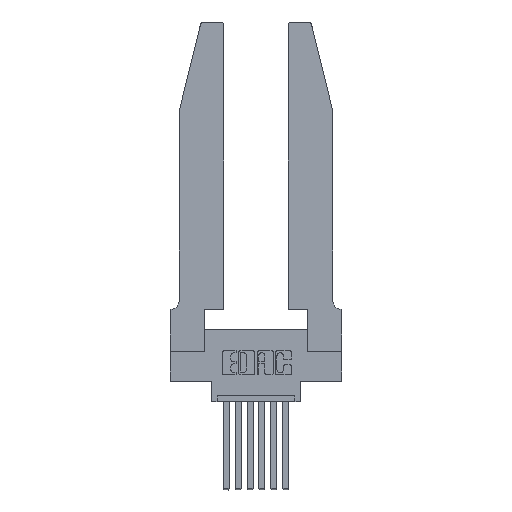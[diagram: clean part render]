
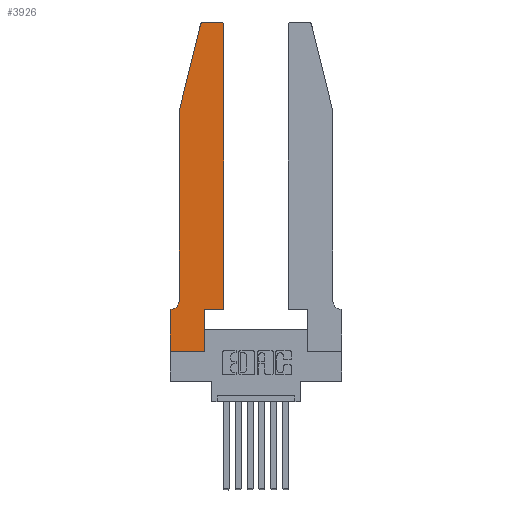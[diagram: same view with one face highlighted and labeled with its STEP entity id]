
A CAD part, top view. The second image highlights one B-rep face of the part: STEP entity #3926.
In plain terms, the highlighted planar face has unit normal (0, 0, 1).
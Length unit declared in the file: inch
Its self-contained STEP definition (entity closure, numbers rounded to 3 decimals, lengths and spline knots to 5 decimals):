
#338 = DIRECTION ( 'NONE',  ( 0., 1., 0. ) ) ;
#465 = ORIENTED_EDGE ( 'NONE', *, *, #9877, .T. ) ;
#530 = CARTESIAN_POINT ( 'NONE',  ( 0.25487, 2.72718, 0.37 ) ) ;
#577 = VECTOR ( 'NONE', #11728, 39.37008 ) ;
#966 = DIRECTION ( 'NONE',  ( 1., 0., 0. ) ) ;
#974 = LINE ( 'NONE', #13848, #13574 ) ;
#1001 = EDGE_LOOP ( 'NONE', ( #7670, #6394, #12149, #5676, #9165, #8569, #6731, #13480, #465, #3043, #10294, #7103 ) ) ;
#1427 = VECTOR ( 'NONE', #12442, 39.37008 ) ;
#1522 = CARTESIAN_POINT ( 'NONE',  ( 0.2865, 0.35, 0.37 ) ) ;
#1587 = VERTEX_POINT ( 'NONE', #5933 ) ;
#1588 = VERTEX_POINT ( 'NONE', #9329 ) ;
#1752 = VERTEX_POINT ( 'NONE', #9555 ) ;
#2120 = AXIS2_PLACEMENT_3D ( 'NONE', #5850, #12301, #6760 ) ;
#2475 = DIRECTION ( 'NONE',  ( 0., 0., 1. ) ) ;
#2496 = CARTESIAN_POINT ( 'NONE',  ( 0.0755, 2., 0.37 ) ) ;
#2511 = CARTESIAN_POINT ( 'NONE',  ( 0.0755, 0.42, 0.37 ) ) ;
#2732 = EDGE_CURVE ( 'NONE', #7018, #10086, #8358, .T. ) ;
#2941 = VERTEX_POINT ( 'NONE', #6949 ) ;
#3043 = ORIENTED_EDGE ( 'NONE', *, *, #10945, .T. ) ;
#3095 = AXIS2_PLACEMENT_3D ( 'NONE', #6288, #5360, #966 ) ;
#3501 = DIRECTION ( 'NONE',  ( 0., -1., 0. ) ) ;
#3838 = CARTESIAN_POINT ( 'NONE',  ( 0.2865, 0.35, 0.37 ) ) ;
#3926 = ADVANCED_FACE ( 'NONE', ( #5076 ), #10661, .T. ) ;
#3950 = VECTOR ( 'NONE', #4097, 39.37008 ) ;
#4097 = DIRECTION ( 'NONE',  ( 0., -1., 0. ) ) ;
#4111 = EDGE_CURVE ( 'NONE', #4497, #4289, #11356, .T. ) ;
#4289 = VERTEX_POINT ( 'NONE', #7799 ) ;
#4497 = VERTEX_POINT ( 'NONE', #2511 ) ;
#4593 = CARTESIAN_POINT ( 'NONE',  ( 0.284, 2.75, 0.37 ) ) ;
#4658 = CARTESIAN_POINT ( 'NONE',  ( 0.4205, 2.72, 0.37 ) ) ;
#4994 = DIRECTION ( 'NONE',  ( -1., 0., 0. ) ) ;
#5076 = FACE_OUTER_BOUND ( 'NONE', #1001, .T. ) ;
#5276 = CARTESIAN_POINT ( 'NONE',  ( 0., 0., 0.37 ) ) ;
#5311 = VECTOR ( 'NONE', #3501, 39.37008 ) ;
#5334 = VERTEX_POINT ( 'NONE', #3838 ) ;
#5360 = DIRECTION ( 'NONE',  ( 0., 0., 1. ) ) ;
#5568 = EDGE_CURVE ( 'NONE', #9836, #9139, #8239, .T. ) ;
#5650 = DIRECTION ( 'NONE',  ( 1., 0., 0. ) ) ;
#5676 = ORIENTED_EDGE ( 'NONE', *, *, #7313, .T. ) ;
#5850 = CARTESIAN_POINT ( 'NONE',  ( 0.0055, 0.42, 0.37 ) ) ;
#5933 = CARTESIAN_POINT ( 'NONE',  ( 0., 0.35, 0.37 ) ) ;
#6051 = VECTOR ( 'NONE', #13645, 39.37008 ) ;
#6288 = CARTESIAN_POINT ( 'NONE',  ( 0., 0.35, 0.37 ) ) ;
#6394 = ORIENTED_EDGE ( 'NONE', *, *, #11330, .T. ) ;
#6709 = DIRECTION ( 'NONE',  ( 1., 0., 0. ) ) ;
#6722 = LINE ( 'NONE', #10276, #1427 ) ;
#6731 = ORIENTED_EDGE ( 'NONE', *, *, #7229, .T. ) ;
#6760 = DIRECTION ( 'NONE',  ( -1., 0., 0. ) ) ;
#6948 = CARTESIAN_POINT ( 'NONE',  ( 0.4205, 2.75, 0.37 ) ) ;
#6949 = CARTESIAN_POINT ( 'NONE',  ( 0., 0., 0.37 ) ) ;
#7018 = VERTEX_POINT ( 'NONE', #8177 ) ;
#7103 = ORIENTED_EDGE ( 'NONE', *, *, #10800, .T. ) ;
#7141 = LINE ( 'NONE', #1522, #8795 ) ;
#7229 = EDGE_CURVE ( 'NONE', #1587, #2941, #9677, .T. ) ;
#7260 = CARTESIAN_POINT ( 'NONE',  ( 0.4505, 0.35, 0.37 ) ) ;
#7313 = EDGE_CURVE ( 'NONE', #1588, #4497, #8182, .T. ) ;
#7504 = VERTEX_POINT ( 'NONE', #530 ) ;
#7670 = ORIENTED_EDGE ( 'NONE', *, *, #5568, .T. ) ;
#7765 = DIRECTION ( 'NONE',  ( 0., 0., 1. ) ) ;
#7799 = CARTESIAN_POINT ( 'NONE',  ( 0.0055, 0.35, 0.37 ) ) ;
#7951 = VECTOR ( 'NONE', #5650, 39.37008 ) ;
#8062 = VECTOR ( 'NONE', #4994, 39.37008 ) ;
#8177 = CARTESIAN_POINT ( 'NONE',  ( 0.4505, 0.35, 0.37 ) ) ;
#8182 = LINE ( 'NONE', #2496, #5311 ) ;
#8239 = LINE ( 'NONE', #11402, #8062 ) ;
#8358 = LINE ( 'NONE', #7260, #577 ) ;
#8474 = CARTESIAN_POINT ( 'NONE',  ( 0.4505, 2.72, 0.37 ) ) ;
#8569 = ORIENTED_EDGE ( 'NONE', *, *, #13128, .T. ) ;
#8607 = CIRCLE ( 'NONE', #12874, 0.03 ) ;
#8795 = VECTOR ( 'NONE', #338, 39.37008 ) ;
#8949 = CARTESIAN_POINT ( 'NONE',  ( 0., 0., 0.37 ) ) ;
#9139 = VERTEX_POINT ( 'NONE', #4593 ) ;
#9165 = ORIENTED_EDGE ( 'NONE', *, *, #4111, .T. ) ;
#9255 = LINE ( 'NONE', #12581, #6051 ) ;
#9329 = CARTESIAN_POINT ( 'NONE',  ( 0.0755, 2., 0.37 ) ) ;
#9555 = CARTESIAN_POINT ( 'NONE',  ( 0.2865, 0., 0.37 ) ) ;
#9677 = LINE ( 'NONE', #5276, #3950 ) ;
#9836 = VERTEX_POINT ( 'NONE', #6948 ) ;
#9877 = EDGE_CURVE ( 'NONE', #1752, #5334, #7141, .T. ) ;
#9920 = AXIS2_PLACEMENT_3D ( 'NONE', #13400, #2475, #6709 ) ;
#9926 = DIRECTION ( 'NONE',  ( 1., 0., 0. ) ) ;
#9951 = CIRCLE ( 'NONE', #9920, 0.03 ) ;
#10086 = VERTEX_POINT ( 'NONE', #8474 ) ;
#10276 = CARTESIAN_POINT ( 'NONE',  ( 0.0755, 0.35, 0.37 ) ) ;
#10286 = EDGE_CURVE ( 'NONE', #2941, #1752, #12412, .T. ) ;
#10294 = ORIENTED_EDGE ( 'NONE', *, *, #2732, .T. ) ;
#10661 = PLANE ( 'NONE',  #3095 ) ;
#10800 = EDGE_CURVE ( 'NONE', #10086, #9836, #8607, .T. ) ;
#10945 = EDGE_CURVE ( 'NONE', #5334, #7018, #974, .T. ) ;
#11330 = EDGE_CURVE ( 'NONE', #9139, #7504, #9951, .T. ) ;
#11356 = CIRCLE ( 'NONE', #2120, 0.07 ) ;
#11402 = CARTESIAN_POINT ( 'NONE',  ( 0.2605, 2.75, 0.37 ) ) ;
#11728 = DIRECTION ( 'NONE',  ( 0., 1., 0. ) ) ;
#12149 = ORIENTED_EDGE ( 'NONE', *, *, #13210, .T. ) ;
#12301 = DIRECTION ( 'NONE',  ( 0., 0., -1. ) ) ;
#12412 = LINE ( 'NONE', #8949, #7951 ) ;
#12442 = DIRECTION ( 'NONE',  ( -1., 0., 0. ) ) ;
#12581 = CARTESIAN_POINT ( 'NONE',  ( 0.0755, 2., 0.37 ) ) ;
#12874 = AXIS2_PLACEMENT_3D ( 'NONE', #4658, #7765, #9926 ) ;
#13128 = EDGE_CURVE ( 'NONE', #4289, #1587, #6722, .T. ) ;
#13210 = EDGE_CURVE ( 'NONE', #7504, #1588, #9255, .T. ) ;
#13400 = CARTESIAN_POINT ( 'NONE',  ( 0.284, 2.72, 0.37 ) ) ;
#13480 = ORIENTED_EDGE ( 'NONE', *, *, #10286, .T. ) ;
#13574 = VECTOR ( 'NONE', #13661, 39.37008 ) ;
#13645 = DIRECTION ( 'NONE',  ( -0.239, -0.971, 0. ) ) ;
#13661 = DIRECTION ( 'NONE',  ( 1., 0., 0. ) ) ;
#13848 = CARTESIAN_POINT ( 'NONE',  ( 0.4505, 0.35, 0.37 ) ) ;
